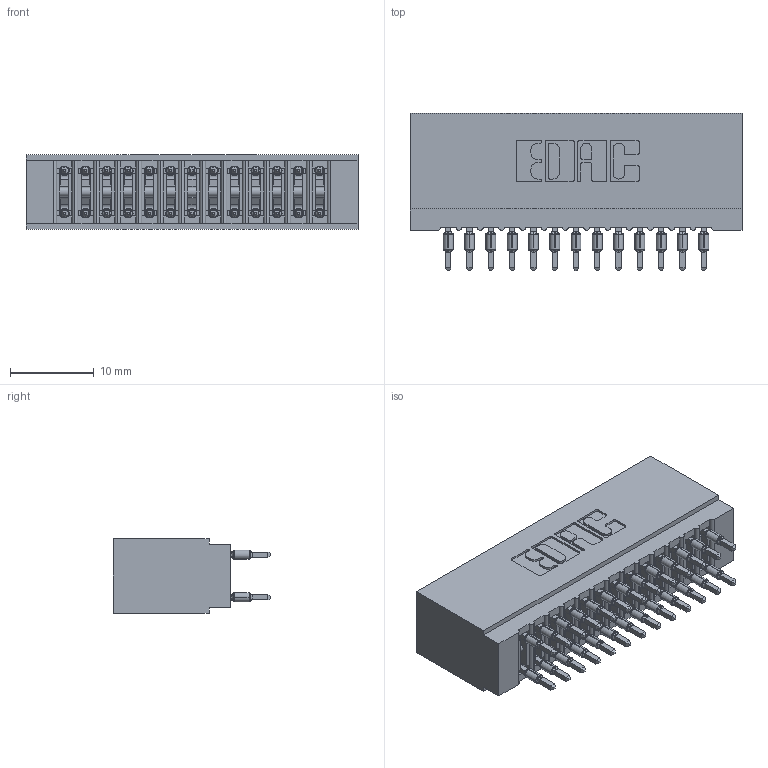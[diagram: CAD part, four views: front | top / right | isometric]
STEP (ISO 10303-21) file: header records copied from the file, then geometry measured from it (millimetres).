
FILE_DESCRIPTION (( 'STEP AP203' ), '1' );
FILE_NAME ('725-026-560-201.STEP', '2026-02-24T17:03:32', ( '' ), ( '' ), 'SwSTEP 2.0', 'SolidWorks 2023', '' );
FILE_SCHEMA (( 'CONFIG_CONTROL_DESIGN' ));
Length unit declared in the file: millimetre
Products named in the file (3): 725-026-560-201; 725 Part_Insulator Option - 01; 745-292-001_560
Assembly tree (27 placements, depth 2):
  725-026-560-201
    725 Part_Insulator Option - 01
    745-292-001_560  x26
Bounding box: 39.62 x 18.8 x 8.89 mm (x, y, z)
Volume: 3384.4 mm3; surface area: 6937.9 mm2
Topology: 27 solids, 27 shells, 2656 faces, 7261 edges, 4614 vertices
Faces by surface type: plane 1381, cylinder 599, bspline 520, torus 156
Entity records: 26132 total; most frequent: CARTESIAN_POINT 5045, ORIENTED_EDGE 4422, DIRECTION 3895, EDGE_CURVE 2211, LINE 1943, VECTOR 1943, VERTEX_POINT 1414, AXIS2_PLACEMENT_3D 976
